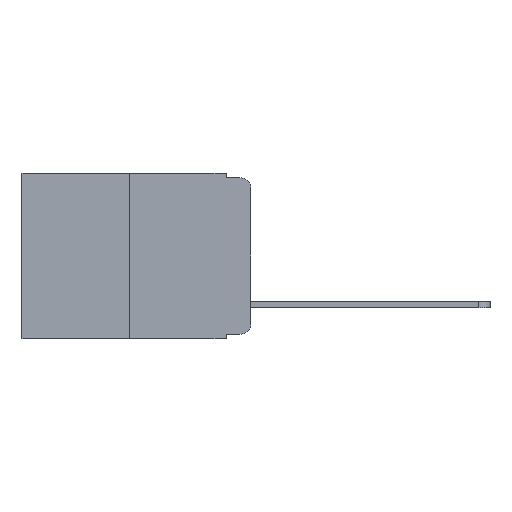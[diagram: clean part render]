
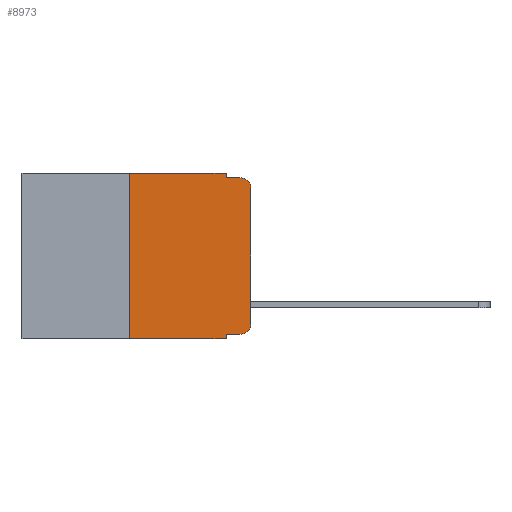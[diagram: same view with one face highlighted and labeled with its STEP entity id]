
A CAD part, left-side view. The second image highlights one B-rep face of the part: STEP entity #8973.
In plain terms, the highlighted planar face has unit normal (-1, 0, 0).
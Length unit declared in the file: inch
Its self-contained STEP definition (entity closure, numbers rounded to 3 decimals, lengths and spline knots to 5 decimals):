
#948 = CARTESIAN_POINT ( 'NONE',  ( 0., 0.02, -0.313 ) ) ;
#1236 = DIRECTION ( 'NONE',  ( -1., 0., 0. ) ) ;
#1318 = VERTEX_POINT ( 'NONE', #18080 ) ;
#1829 = LINE ( 'NONE', #22394, #15477 ) ;
#1948 = DIRECTION ( 'NONE',  ( 0., -1., 0. ) ) ;
#2265 = VECTOR ( 'NONE', #20746, 39.37008 ) ;
#2506 = VERTEX_POINT ( 'NONE', #6507 ) ;
#2732 = CARTESIAN_POINT ( 'NONE',  ( 0., 0.473, 0. ) ) ;
#3302 = DIRECTION ( 'NONE',  ( 0., 0., -1. ) ) ;
#3333 = DIRECTION ( 'NONE',  ( -1., 0., 0. ) ) ;
#4376 = DIRECTION ( 'NONE',  ( 0., -1., 0. ) ) ;
#4569 = ORIENTED_EDGE ( 'NONE', *, *, #8012, .T. ) ;
#4785 = CARTESIAN_POINT ( 'NONE',  ( 0., 0., -0.313 ) ) ;
#4787 = VECTOR ( 'NONE', #1948, 39.37008 ) ;
#4926 = VECTOR ( 'NONE', #4376, 39.37008 ) ;
#5109 = CARTESIAN_POINT ( 'NONE',  ( 0., 0.051, -0.333 ) ) ;
#5138 = CARTESIAN_POINT ( 'NONE',  ( 0., 0.051, 0. ) ) ;
#5367 = EDGE_CURVE ( 'NONE', #15280, #19609, #15106, .T. ) ;
#5427 = EDGE_CURVE ( 'NONE', #11016, #15280, #6001, .T. ) ;
#5477 = ORIENTED_EDGE ( 'NONE', *, *, #5367, .T. ) ;
#5544 = EDGE_CURVE ( 'NONE', #11016, #17212, #11080, .T. ) ;
#5613 = CARTESIAN_POINT ( 'NONE',  ( 0., 0.473, 0. ) ) ;
#5964 = EDGE_CURVE ( 'NONE', #1318, #17148, #7724, .T. ) ;
#6001 = LINE ( 'NONE', #19392, #4787 ) ;
#6089 = AXIS2_PLACEMENT_3D ( 'NONE', #12343, #1236, #13949 ) ;
#6101 = EDGE_CURVE ( 'NONE', #19070, #19821, #7408, .T. ) ;
#6118 = CIRCLE ( 'NONE', #6089, 0.02 ) ;
#6507 = CARTESIAN_POINT ( 'NONE',  ( 0., 0., -0.03 ) ) ;
#6715 = EDGE_CURVE ( 'NONE', #17148, #19070, #7652, .T. ) ;
#7269 = EDGE_CURVE ( 'NONE', #19821, #15171, #9368, .T. ) ;
#7408 = LINE ( 'NONE', #19169, #2265 ) ;
#7508 = DIRECTION ( 'NONE',  ( 1., 0., 0. ) ) ;
#7652 = LINE ( 'NONE', #2732, #20724 ) ;
#7724 = LINE ( 'NONE', #20082, #17608 ) ;
#8012 = EDGE_CURVE ( 'NONE', #2506, #15171, #6118, .T. ) ;
#8220 = EDGE_CURVE ( 'NONE', #19609, #2506, #17214, .T. ) ;
#8458 = VECTOR ( 'NONE', #9750, 39.37008 ) ;
#8973 = ADVANCED_FACE ( 'NONE', ( #9968 ), #15884, .F. ) ;
#9064 = CARTESIAN_POINT ( 'NONE',  ( 0., 0.051, -0.343 ) ) ;
#9368 = LINE ( 'NONE', #14840, #4926 ) ;
#9750 = DIRECTION ( 'NONE',  ( 0., 0., 1. ) ) ;
#9968 = FACE_OUTER_BOUND ( 'NONE', #15731, .T. ) ;
#11016 = VERTEX_POINT ( 'NONE', #5109 ) ;
#11080 = LINE ( 'NONE', #17230, #14861 ) ;
#11669 = ORIENTED_EDGE ( 'NONE', *, *, #6715, .F. ) ;
#12170 = ORIENTED_EDGE ( 'NONE', *, *, #5964, .F. ) ;
#12343 = CARTESIAN_POINT ( 'NONE',  ( 0., 0.02, -0.03 ) ) ;
#12923 = ORIENTED_EDGE ( 'NONE', *, *, #8220, .T. ) ;
#13921 = ORIENTED_EDGE ( 'NONE', *, *, #7269, .F. ) ;
#13949 = DIRECTION ( 'NONE',  ( 0., 0., -1. ) ) ;
#14187 = ORIENTED_EDGE ( 'NONE', *, *, #5544, .F. ) ;
#14490 = DIRECTION ( 'NONE',  ( 0., -1., 0. ) ) ;
#14840 = CARTESIAN_POINT ( 'NONE',  ( 0., 0.051, -0.01 ) ) ;
#14861 = VECTOR ( 'NONE', #15626, 39.37008 ) ;
#14924 = ORIENTED_EDGE ( 'NONE', *, *, #6101, .F. ) ;
#15106 = CIRCLE ( 'NONE', #17108, 0.02 ) ;
#15171 = VERTEX_POINT ( 'NONE', #20279 ) ;
#15280 = VERTEX_POINT ( 'NONE', #20623 ) ;
#15477 = VECTOR ( 'NONE', #14490, 39.37008 ) ;
#15626 = DIRECTION ( 'NONE',  ( 0., 0., -1. ) ) ;
#15731 = EDGE_LOOP ( 'NONE', ( #12923, #4569, #13921, #14924, #11669, #12170, #16955, #14187, #18439, #5477 ) ) ;
#15884 = PLANE ( 'NONE',  #17958 ) ;
#16027 = EDGE_CURVE ( 'NONE', #1318, #17212, #1829, .T. ) ;
#16719 = DIRECTION ( 'NONE',  ( 0., -1., 0. ) ) ;
#16955 = ORIENTED_EDGE ( 'NONE', *, *, #16027, .T. ) ;
#17108 = AXIS2_PLACEMENT_3D ( 'NONE', #948, #3333, #3302 ) ;
#17148 = VERTEX_POINT ( 'NONE', #18654 ) ;
#17212 = VERTEX_POINT ( 'NONE', #9064 ) ;
#17214 = LINE ( 'NONE', #17820, #8458 ) ;
#17230 = CARTESIAN_POINT ( 'NONE',  ( 0., 0.051, 0. ) ) ;
#17608 = VECTOR ( 'NONE', #19996, 39.37008 ) ;
#17820 = CARTESIAN_POINT ( 'NONE',  ( 0., 0., 0. ) ) ;
#17958 = AXIS2_PLACEMENT_3D ( 'NONE', #5613, #7508, #19082 ) ;
#18080 = CARTESIAN_POINT ( 'NONE',  ( 0., 0.25, -0.343 ) ) ;
#18439 = ORIENTED_EDGE ( 'NONE', *, *, #5427, .T. ) ;
#18654 = CARTESIAN_POINT ( 'NONE',  ( 0., 0.25, 0. ) ) ;
#19070 = VERTEX_POINT ( 'NONE', #5138 ) ;
#19082 = DIRECTION ( 'NONE',  ( 0., 0., -1. ) ) ;
#19169 = CARTESIAN_POINT ( 'NONE',  ( 0., 0.051, 0. ) ) ;
#19392 = CARTESIAN_POINT ( 'NONE',  ( 0., 0.051, -0.333 ) ) ;
#19609 = VERTEX_POINT ( 'NONE', #4785 ) ;
#19821 = VERTEX_POINT ( 'NONE', #20587 ) ;
#19996 = DIRECTION ( 'NONE',  ( 0., 0., 1. ) ) ;
#20082 = CARTESIAN_POINT ( 'NONE',  ( 0., 0.25, 0. ) ) ;
#20279 = CARTESIAN_POINT ( 'NONE',  ( 0., 0.02, -0.01 ) ) ;
#20587 = CARTESIAN_POINT ( 'NONE',  ( 0., 0.051, -0.01 ) ) ;
#20623 = CARTESIAN_POINT ( 'NONE',  ( 0., 0.02, -0.333 ) ) ;
#20724 = VECTOR ( 'NONE', #16719, 39.37008 ) ;
#20746 = DIRECTION ( 'NONE',  ( 0., 0., -1. ) ) ;
#22394 = CARTESIAN_POINT ( 'NONE',  ( 0., 0.473, -0.343 ) ) ;
